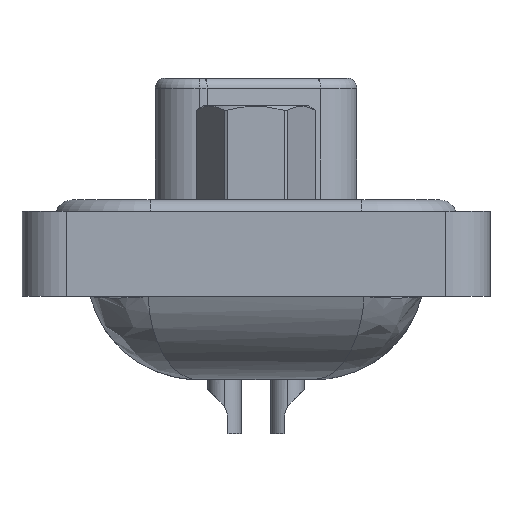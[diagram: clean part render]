
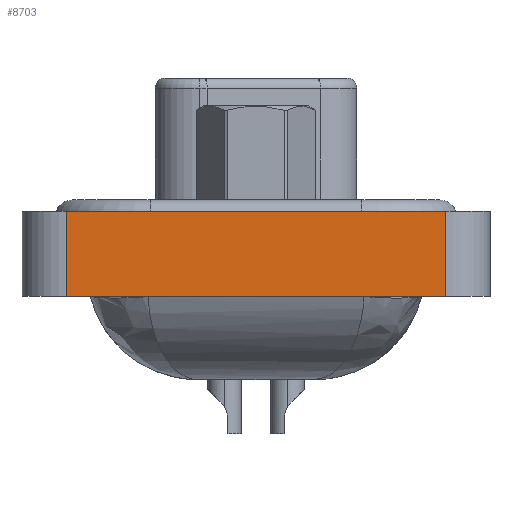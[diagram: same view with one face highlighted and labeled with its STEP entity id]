
A CAD part, left-side view. The second image highlights one B-rep face of the part: STEP entity #8703.
In plain terms, the highlighted planar face has unit normal (-1, 0, 0).
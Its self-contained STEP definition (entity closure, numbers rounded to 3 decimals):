
#203 = DIRECTION ( 'NONE',  ( -1., 0., 0. ) ) ;
#807 = LINE ( 'NONE', #18164, #10945 ) ;
#1390 = DIRECTION ( 'NONE',  ( 0., 0., 1. ) ) ;
#2016 = LINE ( 'NONE', #15347, #26286 ) ;
#2331 = ORIENTED_EDGE ( 'NONE', *, *, #21318, .F. ) ;
#3065 = VERTEX_POINT ( 'NONE', #13913 ) ;
#3282 = CARTESIAN_POINT ( 'NONE',  ( -7.225, -8.55, -3.35 ) ) ;
#3465 = LINE ( 'NONE', #8017, #16338 ) ;
#3959 = CARTESIAN_POINT ( 'NONE',  ( -7.225, -8.55, 0.5 ) ) ;
#5937 = CARTESIAN_POINT ( 'NONE',  ( -7.225, -8.55, -3.35 ) ) ;
#7738 = DIRECTION ( 'NONE',  ( 0., 0., 1. ) ) ;
#8017 = CARTESIAN_POINT ( 'NONE',  ( -7.225, 8.55, -3.35 ) ) ;
#8703 = ADVANCED_FACE ( 'NONE', ( #13273 ), #12988, .T. ) ;
#9135 = CARTESIAN_POINT ( 'NONE',  ( -7.225, -8.55, -3.35 ) ) ;
#9900 = AXIS2_PLACEMENT_3D ( 'NONE', #9135, #203, #15384 ) ;
#10599 = EDGE_CURVE ( 'NONE', #13102, #19887, #20867, .T. ) ;
#10945 = VECTOR ( 'NONE', #18447, 1000. ) ;
#11707 = ORIENTED_EDGE ( 'NONE', *, *, #14049, .F. ) ;
#12988 = PLANE ( 'NONE',  #9900 ) ;
#13102 = VERTEX_POINT ( 'NONE', #3282 ) ;
#13273 = FACE_OUTER_BOUND ( 'NONE', #22043, .T. ) ;
#13913 = CARTESIAN_POINT ( 'NONE',  ( -7.225, 8.55, -3.35 ) ) ;
#14049 = EDGE_CURVE ( 'NONE', #19602, #19887, #807, .T. ) ;
#14534 = VECTOR ( 'NONE', #1390, 1000. ) ;
#15347 = CARTESIAN_POINT ( 'NONE',  ( -7.225, -8.55, -3.35 ) ) ;
#15384 = DIRECTION ( 'NONE',  ( 0., 0., 1. ) ) ;
#16338 = VECTOR ( 'NONE', #7738, 1000. ) ;
#18164 = CARTESIAN_POINT ( 'NONE',  ( -7.225, -8.55, 0.5 ) ) ;
#18447 = DIRECTION ( 'NONE',  ( 0., -1., 0. ) ) ;
#19602 = VERTEX_POINT ( 'NONE', #24418 ) ;
#19887 = VERTEX_POINT ( 'NONE', #3959 ) ;
#20867 = LINE ( 'NONE', #5937, #14534 ) ;
#21318 = EDGE_CURVE ( 'NONE', #3065, #19602, #3465, .T. ) ;
#21443 = ORIENTED_EDGE ( 'NONE', *, *, #10599, .T. ) ;
#22043 = EDGE_LOOP ( 'NONE', ( #21443, #11707, #2331, #25422 ) ) ;
#23406 = EDGE_CURVE ( 'NONE', #3065, #13102, #2016, .T. ) ;
#24418 = CARTESIAN_POINT ( 'NONE',  ( -7.225, 8.55, 0.5 ) ) ;
#25422 = ORIENTED_EDGE ( 'NONE', *, *, #23406, .T. ) ;
#26131 = DIRECTION ( 'NONE',  ( 0., -1., 0. ) ) ;
#26286 = VECTOR ( 'NONE', #26131, 1000. ) ;
